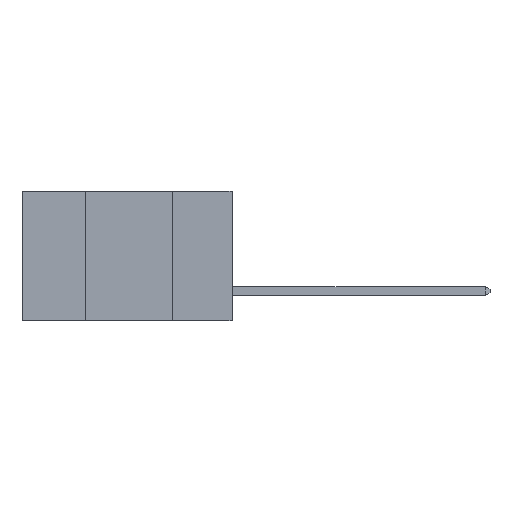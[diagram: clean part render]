
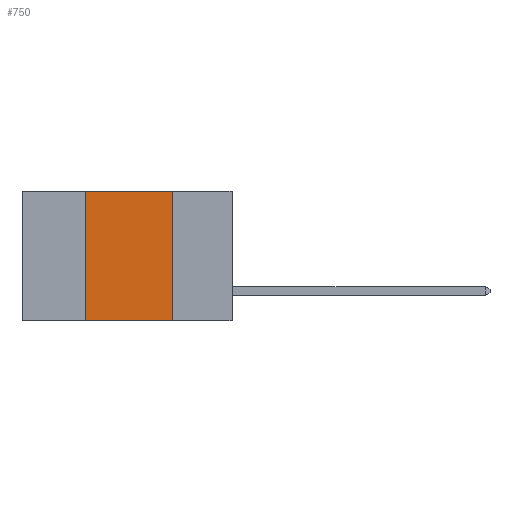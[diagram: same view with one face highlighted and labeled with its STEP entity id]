
A CAD part, left-side view. The second image highlights one B-rep face of the part: STEP entity #750.
In plain terms, the highlighted planar face has unit normal (-1, 0, 0).
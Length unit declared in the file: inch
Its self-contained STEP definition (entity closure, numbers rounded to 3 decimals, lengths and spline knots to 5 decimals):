
#378 = DIRECTION ( 'NONE',  ( 0., -1., 0. ) ) ;
#421 = FACE_OUTER_BOUND ( 'NONE', #8985, .T. ) ;
#750 = ADVANCED_FACE ( 'NONE', ( #421 ), #6665, .F. ) ;
#1170 = LINE ( 'NONE', #9075, #4173 ) ;
#2157 = EDGE_CURVE ( 'NONE', #5758, #12109, #15030, .T. ) ;
#2251 = CARTESIAN_POINT ( 'NONE',  ( 0., 0.42, -0.37 ) ) ;
#4156 = CARTESIAN_POINT ( 'NONE',  ( 0., 0.42, 0. ) ) ;
#4173 = VECTOR ( 'NONE', #10279, 39.37008 ) ;
#4887 = EDGE_CURVE ( 'NONE', #5458, #12317, #14237, .T. ) ;
#5458 = VERTEX_POINT ( 'NONE', #4156 ) ;
#5464 = CARTESIAN_POINT ( 'NONE',  ( 0., 0.17, -0.37 ) ) ;
#5511 = CARTESIAN_POINT ( 'NONE',  ( 0., 0.6, 0. ) ) ;
#5758 = VERTEX_POINT ( 'NONE', #2251 ) ;
#5781 = CARTESIAN_POINT ( 'NONE',  ( 0., 0.6, 0. ) ) ;
#5844 = DIRECTION ( 'NONE',  ( 0., 0., -1. ) ) ;
#6022 = DIRECTION ( 'NONE',  ( 1., 0., 0. ) ) ;
#6653 = DIRECTION ( 'NONE',  ( 0., 0., 1. ) ) ;
#6665 = PLANE ( 'NONE',  #14102 ) ;
#7899 = CARTESIAN_POINT ( 'NONE',  ( 0., 0.42, 0. ) ) ;
#8036 = LINE ( 'NONE', #7899, #10850 ) ;
#8227 = CARTESIAN_POINT ( 'NONE',  ( 0., 0.6, -0.37 ) ) ;
#8977 = VECTOR ( 'NONE', #11842, 39.37008 ) ;
#8985 = EDGE_LOOP ( 'NONE', ( #14083, #11854, #11998, #11775 ) ) ;
#9075 = CARTESIAN_POINT ( 'NONE',  ( 0., 0.17, 0. ) ) ;
#9617 = CARTESIAN_POINT ( 'NONE',  ( 0., 0.17, 0. ) ) ;
#10279 = DIRECTION ( 'NONE',  ( 0., 0., -1. ) ) ;
#10506 = EDGE_CURVE ( 'NONE', #5758, #5458, #8036, .T. ) ;
#10509 = EDGE_CURVE ( 'NONE', #12317, #12109, #1170, .T. ) ;
#10850 = VECTOR ( 'NONE', #6653, 39.37008 ) ;
#11022 = VECTOR ( 'NONE', #378, 39.37008 ) ;
#11775 = ORIENTED_EDGE ( 'NONE', *, *, #2157, .T. ) ;
#11842 = DIRECTION ( 'NONE',  ( 0., -1., 0. ) ) ;
#11854 = ORIENTED_EDGE ( 'NONE', *, *, #4887, .F. ) ;
#11998 = ORIENTED_EDGE ( 'NONE', *, *, #10506, .F. ) ;
#12109 = VERTEX_POINT ( 'NONE', #5464 ) ;
#12317 = VERTEX_POINT ( 'NONE', #9617 ) ;
#14083 = ORIENTED_EDGE ( 'NONE', *, *, #10509, .F. ) ;
#14102 = AXIS2_PLACEMENT_3D ( 'NONE', #5781, #6022, #5844 ) ;
#14237 = LINE ( 'NONE', #5511, #11022 ) ;
#15030 = LINE ( 'NONE', #8227, #8977 ) ;
